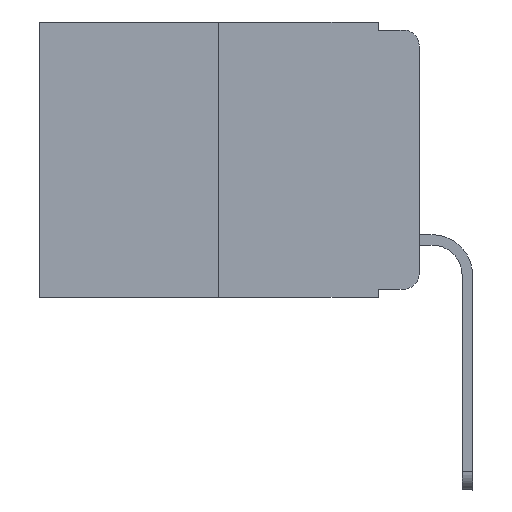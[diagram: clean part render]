
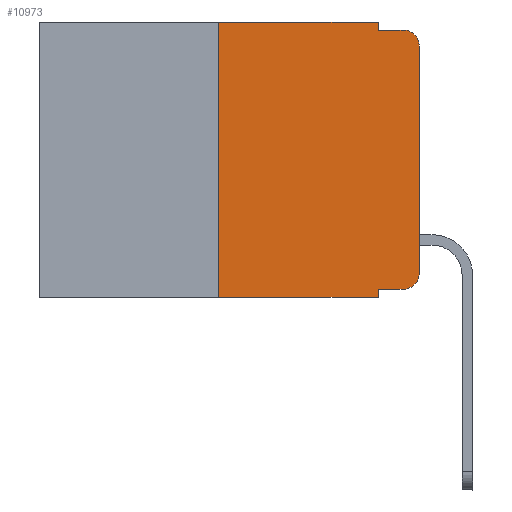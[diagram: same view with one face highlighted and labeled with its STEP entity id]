
A CAD part, left-side view. The second image highlights one B-rep face of the part: STEP entity #10973.
In plain terms, the highlighted planar face has unit normal (-1, 0, 0).
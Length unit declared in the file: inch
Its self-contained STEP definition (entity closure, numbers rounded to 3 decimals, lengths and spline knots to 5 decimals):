
#726 = EDGE_CURVE ( 'NONE', #15576, #16984, #4184, .T. ) ;
#738 = DIRECTION ( 'NONE',  ( 0., -1., 0. ) ) ;
#1936 = CARTESIAN_POINT ( 'NONE',  ( 0., 0.051, -0.333 ) ) ;
#2142 = CARTESIAN_POINT ( 'NONE',  ( 0., 0.051, 0. ) ) ;
#2169 = DIRECTION ( 'NONE',  ( 0., -1., 0. ) ) ;
#2502 = DIRECTION ( 'NONE',  ( 1., 0., 0. ) ) ;
#2594 = DIRECTION ( 'NONE',  ( 0., -1., 0. ) ) ;
#2647 = EDGE_CURVE ( 'NONE', #20137, #9046, #6290, .T. ) ;
#2717 = CIRCLE ( 'NONE', #19004, 0.02 ) ;
#2826 = LINE ( 'NONE', #18031, #7942 ) ;
#2946 = VERTEX_POINT ( 'NONE', #9382 ) ;
#3159 = CARTESIAN_POINT ( 'NONE',  ( 0., 0., -0.03 ) ) ;
#3214 = CARTESIAN_POINT ( 'NONE',  ( 0., 0.02, -0.03 ) ) ;
#3372 = VECTOR ( 'NONE', #20463, 39.37008 ) ;
#3449 = EDGE_CURVE ( 'NONE', #11245, #16132, #19983, .T. ) ;
#4119 = VECTOR ( 'NONE', #13815, 39.37008 ) ;
#4169 = PLANE ( 'NONE',  #6773 ) ;
#4184 = LINE ( 'NONE', #10984, #19534 ) ;
#4350 = CARTESIAN_POINT ( 'NONE',  ( 0., 0.02, -0.313 ) ) ;
#4898 = DIRECTION ( 'NONE',  ( 0., 0., -1. ) ) ;
#5711 = CARTESIAN_POINT ( 'NONE',  ( 0., 0.473, 0. ) ) ;
#6060 = CARTESIAN_POINT ( 'NONE',  ( 0., 0.051, -0.333 ) ) ;
#6290 = LINE ( 'NONE', #14624, #16348 ) ;
#6773 = AXIS2_PLACEMENT_3D ( 'NONE', #10967, #2502, #9295 ) ;
#6918 = LINE ( 'NONE', #8489, #3372 ) ;
#7942 = VECTOR ( 'NONE', #2594, 39.37008 ) ;
#7987 = ORIENTED_EDGE ( 'NONE', *, *, #20754, .T. ) ;
#8153 = CARTESIAN_POINT ( 'NONE',  ( 0., 0.02, -0.333 ) ) ;
#8489 = CARTESIAN_POINT ( 'NONE',  ( 0., 0.051, -0.01 ) ) ;
#8613 = ORIENTED_EDGE ( 'NONE', *, *, #14169, .T. ) ;
#8916 = LINE ( 'NONE', #2142, #4119 ) ;
#9046 = VERTEX_POINT ( 'NONE', #17696 ) ;
#9058 = LINE ( 'NONE', #5711, #17541 ) ;
#9295 = DIRECTION ( 'NONE',  ( 0., 0., -1. ) ) ;
#9382 = CARTESIAN_POINT ( 'NONE',  ( 0., 0.02, -0.01 ) ) ;
#9389 = ORIENTED_EDGE ( 'NONE', *, *, #10951, .T. ) ;
#10951 = EDGE_CURVE ( 'NONE', #11245, #11448, #21260, .T. ) ;
#10967 = CARTESIAN_POINT ( 'NONE',  ( 0., 0.473, 0. ) ) ;
#10973 = ADVANCED_FACE ( 'NONE', ( #19362 ), #4169, .F. ) ;
#10984 = CARTESIAN_POINT ( 'NONE',  ( 0., 0., 0. ) ) ;
#11054 = ORIENTED_EDGE ( 'NONE', *, *, #18130, .F. ) ;
#11153 = DIRECTION ( 'NONE',  ( -1., 0., 0. ) ) ;
#11245 = VERTEX_POINT ( 'NONE', #1936 ) ;
#11327 = DIRECTION ( 'NONE',  ( 0., 0., 1. ) ) ;
#11448 = VERTEX_POINT ( 'NONE', #8153 ) ;
#12596 = CARTESIAN_POINT ( 'NONE',  ( 0., 0.051, -0.01 ) ) ;
#13479 = CARTESIAN_POINT ( 'NONE',  ( 0., 0.051, -0.343 ) ) ;
#13558 = CARTESIAN_POINT ( 'NONE',  ( 0., 0.25, -0.343 ) ) ;
#13815 = DIRECTION ( 'NONE',  ( 0., 0., -1. ) ) ;
#14169 = EDGE_CURVE ( 'NONE', #20137, #16132, #2826, .T. ) ;
#14624 = CARTESIAN_POINT ( 'NONE',  ( 0., 0.25, 0. ) ) ;
#14793 = DIRECTION ( 'NONE',  ( 0., 0., -1. ) ) ;
#14834 = CARTESIAN_POINT ( 'NONE',  ( 0., 0., -0.313 ) ) ;
#15005 = ORIENTED_EDGE ( 'NONE', *, *, #21295, .T. ) ;
#15278 = VECTOR ( 'NONE', #14793, 39.37008 ) ;
#15576 = VERTEX_POINT ( 'NONE', #14834 ) ;
#16056 = CARTESIAN_POINT ( 'NONE',  ( 0., 0.051, 0. ) ) ;
#16132 = VERTEX_POINT ( 'NONE', #13479 ) ;
#16348 = VECTOR ( 'NONE', #21371, 39.37008 ) ;
#16984 = VERTEX_POINT ( 'NONE', #3159 ) ;
#17135 = VERTEX_POINT ( 'NONE', #12596 ) ;
#17268 = CIRCLE ( 'NONE', #19763, 0.02 ) ;
#17541 = VECTOR ( 'NONE', #2169, 39.37008 ) ;
#17696 = CARTESIAN_POINT ( 'NONE',  ( 0., 0.25, 0. ) ) ;
#17977 = ORIENTED_EDGE ( 'NONE', *, *, #19213, .F. ) ;
#17995 = CARTESIAN_POINT ( 'NONE',  ( 0., 0.051, 0. ) ) ;
#18031 = CARTESIAN_POINT ( 'NONE',  ( 0., 0.473, -0.343 ) ) ;
#18130 = EDGE_CURVE ( 'NONE', #18586, #17135, #8916, .T. ) ;
#18586 = VERTEX_POINT ( 'NONE', #16056 ) ;
#18749 = ORIENTED_EDGE ( 'NONE', *, *, #726, .T. ) ;
#18964 = EDGE_CURVE ( 'NONE', #9046, #18586, #9058, .T. ) ;
#19004 = AXIS2_PLACEMENT_3D ( 'NONE', #4350, #11153, #21334 ) ;
#19200 = ORIENTED_EDGE ( 'NONE', *, *, #18964, .F. ) ;
#19213 = EDGE_CURVE ( 'NONE', #17135, #2946, #6918, .T. ) ;
#19362 = FACE_OUTER_BOUND ( 'NONE', #21263, .T. ) ;
#19534 = VECTOR ( 'NONE', #11327, 39.37008 ) ;
#19763 = AXIS2_PLACEMENT_3D ( 'NONE', #3214, #20414, #4898 ) ;
#19983 = LINE ( 'NONE', #17995, #15278 ) ;
#20137 = VERTEX_POINT ( 'NONE', #13558 ) ;
#20241 = VECTOR ( 'NONE', #738, 39.37008 ) ;
#20414 = DIRECTION ( 'NONE',  ( -1., 0., 0. ) ) ;
#20463 = DIRECTION ( 'NONE',  ( 0., -1., 0. ) ) ;
#20530 = ORIENTED_EDGE ( 'NONE', *, *, #3449, .F. ) ;
#20754 = EDGE_CURVE ( 'NONE', #11448, #15576, #2717, .T. ) ;
#21260 = LINE ( 'NONE', #6060, #20241 ) ;
#21263 = EDGE_LOOP ( 'NONE', ( #18749, #15005, #17977, #11054, #19200, #21449, #8613, #20530, #9389, #7987 ) ) ;
#21295 = EDGE_CURVE ( 'NONE', #16984, #2946, #17268, .T. ) ;
#21334 = DIRECTION ( 'NONE',  ( 0., 0., -1. ) ) ;
#21371 = DIRECTION ( 'NONE',  ( 0., 0., 1. ) ) ;
#21449 = ORIENTED_EDGE ( 'NONE', *, *, #2647, .F. ) ;
